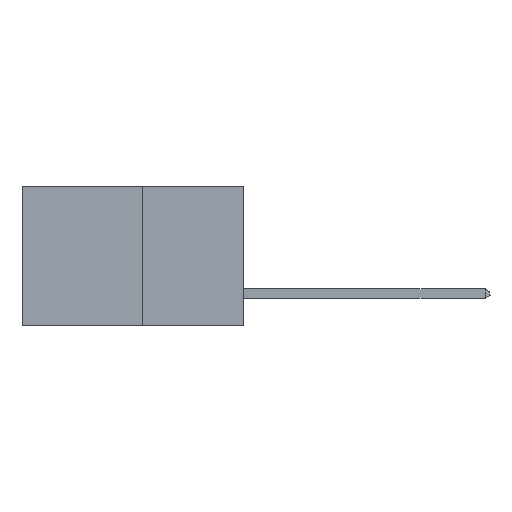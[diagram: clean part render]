
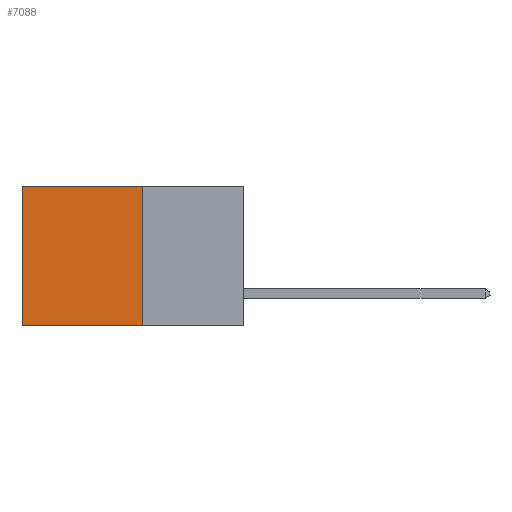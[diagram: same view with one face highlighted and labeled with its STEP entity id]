
A CAD part, left-side view. The second image highlights one B-rep face of the part: STEP entity #7088.
In plain terms, the highlighted planar face has unit normal (-1, 0, 0).
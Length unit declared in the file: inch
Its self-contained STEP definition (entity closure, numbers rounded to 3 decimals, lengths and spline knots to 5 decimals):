
#315 = VERTEX_POINT ( 'NONE', #1088 ) ;
#776 = LINE ( 'NONE', #11022, #5303 ) ;
#1088 = CARTESIAN_POINT ( 'NONE',  ( 0.277, 0.27, -0.37 ) ) ;
#1461 = AXIS2_PLACEMENT_3D ( 'NONE', #2642, #5284, #3548 ) ;
#1710 = EDGE_LOOP ( 'NONE', ( #8723, #5334, #8590, #7592 ) ) ;
#2536 = DIRECTION ( 'NONE',  ( 0., 1., 0. ) ) ;
#2642 = CARTESIAN_POINT ( 'NONE',  ( 0.277, 0.27, -0.37 ) ) ;
#3548 = DIRECTION ( 'NONE',  ( 0., 0., -1. ) ) ;
#4151 = VECTOR ( 'NONE', #9816, 39.37008 ) ;
#4301 = CARTESIAN_POINT ( 'NONE',  ( 0.277, 0.27, -0.37 ) ) ;
#4479 = CARTESIAN_POINT ( 'NONE',  ( 0.277, 0.59, -0.37 ) ) ;
#5076 = CARTESIAN_POINT ( 'NONE',  ( 0.277, 0.27, 0. ) ) ;
#5284 = DIRECTION ( 'NONE',  ( 1., 0., 0. ) ) ;
#5303 = VECTOR ( 'NONE', #5690, 39.37008 ) ;
#5334 = ORIENTED_EDGE ( 'NONE', *, *, #9805, .F. ) ;
#5503 = VERTEX_POINT ( 'NONE', #5076 ) ;
#5690 = DIRECTION ( 'NONE',  ( 0., 1., 0. ) ) ;
#5759 = EDGE_CURVE ( 'NONE', #5503, #315, #8852, .T. ) ;
#5929 = CARTESIAN_POINT ( 'NONE',  ( 0.277, 0.59, -0.37 ) ) ;
#6457 = VECTOR ( 'NONE', #8090, 39.37008 ) ;
#6769 = EDGE_CURVE ( 'NONE', #5503, #7183, #776, .T. ) ;
#6801 = LINE ( 'NONE', #4479, #4151 ) ;
#7088 = ADVANCED_FACE ( 'NONE', ( #9093 ), #7996, .F. ) ;
#7167 = CARTESIAN_POINT ( 'NONE',  ( 0.277, 0.27, -0.37 ) ) ;
#7183 = VERTEX_POINT ( 'NONE', #8159 ) ;
#7592 = ORIENTED_EDGE ( 'NONE', *, *, #6769, .T. ) ;
#7996 = PLANE ( 'NONE',  #1461 ) ;
#8090 = DIRECTION ( 'NONE',  ( 0., 0., -1. ) ) ;
#8159 = CARTESIAN_POINT ( 'NONE',  ( 0.277, 0.59, 0. ) ) ;
#8590 = ORIENTED_EDGE ( 'NONE', *, *, #5759, .F. ) ;
#8723 = ORIENTED_EDGE ( 'NONE', *, *, #11296, .T. ) ;
#8852 = LINE ( 'NONE', #7167, #6457 ) ;
#9093 = FACE_OUTER_BOUND ( 'NONE', #1710, .T. ) ;
#9805 = EDGE_CURVE ( 'NONE', #315, #10329, #11567, .T. ) ;
#9816 = DIRECTION ( 'NONE',  ( 0., 0., -1. ) ) ;
#10329 = VERTEX_POINT ( 'NONE', #5929 ) ;
#11022 = CARTESIAN_POINT ( 'NONE',  ( 0.277, 0.27, 0. ) ) ;
#11026 = VECTOR ( 'NONE', #2536, 39.37008 ) ;
#11296 = EDGE_CURVE ( 'NONE', #7183, #10329, #6801, .T. ) ;
#11567 = LINE ( 'NONE', #4301, #11026 ) ;
